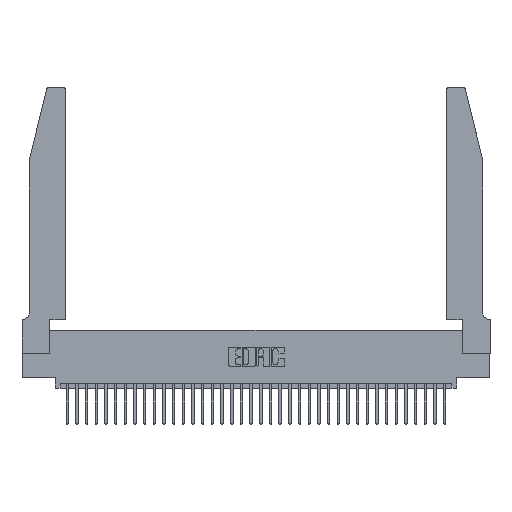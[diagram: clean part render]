
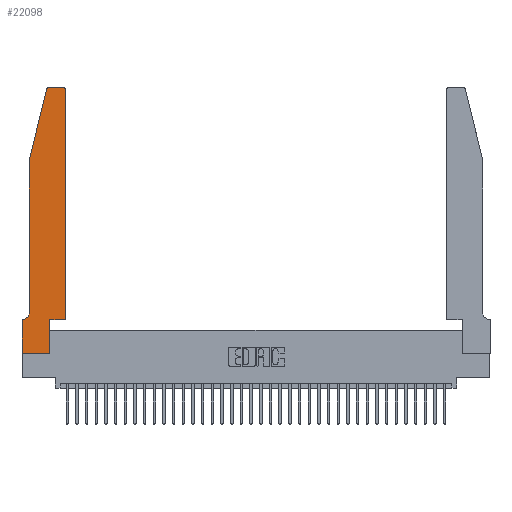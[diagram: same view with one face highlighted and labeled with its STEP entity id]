
A CAD part, top view. The second image highlights one B-rep face of the part: STEP entity #22098.
In plain terms, the highlighted planar face has unit normal (0, 0, 1).
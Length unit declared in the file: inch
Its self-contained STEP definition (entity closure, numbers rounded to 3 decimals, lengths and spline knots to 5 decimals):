
#383 = ORIENTED_EDGE ( 'NONE', *, *, #22573, .T. ) ;
#684 = EDGE_CURVE ( 'NONE', #2675, #20622, #16501, .T. ) ;
#1224 = VERTEX_POINT ( 'NONE', #18128 ) ;
#1583 = EDGE_CURVE ( 'NONE', #23767, #16302, #4445, .T. ) ;
#1666 = DIRECTION ( 'NONE',  ( -1., 0., 0. ) ) ;
#2594 = LINE ( 'NONE', #25634, #26384 ) ;
#2675 = VERTEX_POINT ( 'NONE', #5836 ) ;
#3326 = AXIS2_PLACEMENT_3D ( 'NONE', #4689, #27017, #1666 ) ;
#3863 = CARTESIAN_POINT ( 'NONE',  ( 0., 0.35, 0.37 ) ) ;
#4128 = CARTESIAN_POINT ( 'NONE',  ( 0.0755, 0.35, 0.37 ) ) ;
#4315 = AXIS2_PLACEMENT_3D ( 'NONE', #22122, #36177, #19296 ) ;
#4445 = CIRCLE ( 'NONE', #4315, 0.03 ) ;
#4455 = LINE ( 'NONE', #4128, #26075 ) ;
#4612 = ORIENTED_EDGE ( 'NONE', *, *, #11378, .T. ) ;
#4689 = CARTESIAN_POINT ( 'NONE',  ( 0.0055, 0.42, 0.37 ) ) ;
#5836 = CARTESIAN_POINT ( 'NONE',  ( 0.4505, 0.35, 0.37 ) ) ;
#6321 = DIRECTION ( 'NONE',  ( -0.239, -0.971, 0. ) ) ;
#6413 = ORIENTED_EDGE ( 'NONE', *, *, #23465, .T. ) ;
#6434 = CARTESIAN_POINT ( 'NONE',  ( 0.2865, 0.35, 0.37 ) ) ;
#6522 = EDGE_CURVE ( 'NONE', #20622, #33442, #31228, .T. ) ;
#6792 = CARTESIAN_POINT ( 'NONE',  ( 0.0755, 2., 0.37 ) ) ;
#7374 = LINE ( 'NONE', #18657, #24189 ) ;
#8172 = DIRECTION ( 'NONE',  ( -1., 0., 0. ) ) ;
#8291 = VECTOR ( 'NONE', #10753, 39.37008 ) ;
#9254 = ORIENTED_EDGE ( 'NONE', *, *, #1583, .T. ) ;
#9983 = CARTESIAN_POINT ( 'NONE',  ( 0.4505, 2.72, 0.37 ) ) ;
#10243 = DIRECTION ( 'NONE',  ( 0., 1., 0. ) ) ;
#10327 = DIRECTION ( 'NONE',  ( 1., 0., 0. ) ) ;
#10489 = LINE ( 'NONE', #28172, #11786 ) ;
#10753 = DIRECTION ( 'NONE',  ( 1., 0., 0. ) ) ;
#11176 = PLANE ( 'NONE',  #29555 ) ;
#11275 = VERTEX_POINT ( 'NONE', #21502 ) ;
#11378 = EDGE_CURVE ( 'NONE', #16302, #18760, #2594, .T. ) ;
#11564 = CARTESIAN_POINT ( 'NONE',  ( 0., 0., 0.37 ) ) ;
#11629 = CARTESIAN_POINT ( 'NONE',  ( 0.284, 2.75, 0.37 ) ) ;
#11786 = VECTOR ( 'NONE', #30849, 39.37008 ) ;
#12093 = EDGE_CURVE ( 'NONE', #14893, #27153, #23730, .T. ) ;
#12177 = EDGE_CURVE ( 'NONE', #27153, #2675, #17992, .T. ) ;
#12206 = ORIENTED_EDGE ( 'NONE', *, *, #25421, .T. ) ;
#14321 = ORIENTED_EDGE ( 'NONE', *, *, #12177, .T. ) ;
#14669 = ORIENTED_EDGE ( 'NONE', *, *, #35625, .T. ) ;
#14893 = VERTEX_POINT ( 'NONE', #35311 ) ;
#15030 = ORIENTED_EDGE ( 'NONE', *, *, #19410, .T. ) ;
#16160 = CARTESIAN_POINT ( 'NONE',  ( 0.4505, 0.35, 0.37 ) ) ;
#16302 = VERTEX_POINT ( 'NONE', #30045 ) ;
#16441 = VECTOR ( 'NONE', #31207, 39.37008 ) ;
#16501 = LINE ( 'NONE', #16160, #34468 ) ;
#17051 = CARTESIAN_POINT ( 'NONE',  ( 0.2605, 2.75, 0.37 ) ) ;
#17063 = EDGE_LOOP ( 'NONE', ( #14669, #9254, #4612, #12206, #6413, #383, #15030, #34356, #17687, #14321, #23517, #34891 ) ) ;
#17235 = LINE ( 'NONE', #11564, #16441 ) ;
#17679 = LINE ( 'NONE', #17051, #34008 ) ;
#17687 = ORIENTED_EDGE ( 'NONE', *, *, #12093, .T. ) ;
#17992 = LINE ( 'NONE', #24804, #8291 ) ;
#18128 = CARTESIAN_POINT ( 'NONE',  ( 0., 0., 0.37 ) ) ;
#18170 = FACE_OUTER_BOUND ( 'NONE', #17063, .T. ) ;
#18657 = CARTESIAN_POINT ( 'NONE',  ( 0.0755, 2., 0.37 ) ) ;
#18760 = VERTEX_POINT ( 'NONE', #6792 ) ;
#18912 = CARTESIAN_POINT ( 'NONE',  ( 0.4205, 2.75, 0.37 ) ) ;
#19110 = CARTESIAN_POINT ( 'NONE',  ( 0.4205, 2.72, 0.37 ) ) ;
#19264 = DIRECTION ( 'NONE',  ( 0., 1., 0. ) ) ;
#19296 = DIRECTION ( 'NONE',  ( 1., 0., 0. ) ) ;
#19410 = EDGE_CURVE ( 'NONE', #24110, #1224, #10489, .T. ) ;
#19455 = DIRECTION ( 'NONE',  ( 0., 0., 1. ) ) ;
#20431 = AXIS2_PLACEMENT_3D ( 'NONE', #19110, #32601, #10327 ) ;
#20622 = VERTEX_POINT ( 'NONE', #9983 ) ;
#21502 = CARTESIAN_POINT ( 'NONE',  ( 0.0755, 0.42, 0.37 ) ) ;
#22098 = ADVANCED_FACE ( 'NONE', ( #18170 ), #11176, .T. ) ;
#22122 = CARTESIAN_POINT ( 'NONE',  ( 0.284, 2.72, 0.37 ) ) ;
#22573 = EDGE_CURVE ( 'NONE', #26442, #24110, #4455, .T. ) ;
#22598 = CIRCLE ( 'NONE', #3326, 0.07 ) ;
#23229 = EDGE_CURVE ( 'NONE', #1224, #14893, #17235, .T. ) ;
#23465 = EDGE_CURVE ( 'NONE', #11275, #26442, #22598, .T. ) ;
#23517 = ORIENTED_EDGE ( 'NONE', *, *, #684, .T. ) ;
#23730 = LINE ( 'NONE', #27100, #26775 ) ;
#23767 = VERTEX_POINT ( 'NONE', #11629 ) ;
#23927 = DIRECTION ( 'NONE',  ( -1., 0., 0. ) ) ;
#24110 = VERTEX_POINT ( 'NONE', #3863 ) ;
#24189 = VECTOR ( 'NONE', #24199, 39.37008 ) ;
#24199 = DIRECTION ( 'NONE',  ( 0., -1., 0. ) ) ;
#24804 = CARTESIAN_POINT ( 'NONE',  ( 0.4505, 0.35, 0.37 ) ) ;
#25421 = EDGE_CURVE ( 'NONE', #18760, #11275, #7374, .T. ) ;
#25634 = CARTESIAN_POINT ( 'NONE',  ( 0.0755, 2., 0.37 ) ) ;
#26075 = VECTOR ( 'NONE', #23927, 39.37008 ) ;
#26384 = VECTOR ( 'NONE', #6321, 39.37008 ) ;
#26442 = VERTEX_POINT ( 'NONE', #34064 ) ;
#26775 = VECTOR ( 'NONE', #10243, 39.37008 ) ;
#27017 = DIRECTION ( 'NONE',  ( 0., 0., -1. ) ) ;
#27100 = CARTESIAN_POINT ( 'NONE',  ( 0.2865, 0.35, 0.37 ) ) ;
#27153 = VERTEX_POINT ( 'NONE', #6434 ) ;
#28172 = CARTESIAN_POINT ( 'NONE',  ( 0., 0., 0.37 ) ) ;
#29555 = AXIS2_PLACEMENT_3D ( 'NONE', #36216, #19455, #30713 ) ;
#30045 = CARTESIAN_POINT ( 'NONE',  ( 0.25487, 2.72718, 0.37 ) ) ;
#30713 = DIRECTION ( 'NONE',  ( 1., 0., 0. ) ) ;
#30849 = DIRECTION ( 'NONE',  ( 0., -1., 0. ) ) ;
#31207 = DIRECTION ( 'NONE',  ( 1., 0., 0. ) ) ;
#31228 = CIRCLE ( 'NONE', #20431, 0.03 ) ;
#32601 = DIRECTION ( 'NONE',  ( 0., 0., 1. ) ) ;
#33442 = VERTEX_POINT ( 'NONE', #18912 ) ;
#34008 = VECTOR ( 'NONE', #8172, 39.37008 ) ;
#34064 = CARTESIAN_POINT ( 'NONE',  ( 0.0055, 0.35, 0.37 ) ) ;
#34356 = ORIENTED_EDGE ( 'NONE', *, *, #23229, .T. ) ;
#34468 = VECTOR ( 'NONE', #19264, 39.37008 ) ;
#34891 = ORIENTED_EDGE ( 'NONE', *, *, #6522, .T. ) ;
#35311 = CARTESIAN_POINT ( 'NONE',  ( 0.2865, 0., 0.37 ) ) ;
#35625 = EDGE_CURVE ( 'NONE', #33442, #23767, #17679, .T. ) ;
#36177 = DIRECTION ( 'NONE',  ( 0., 0., 1. ) ) ;
#36216 = CARTESIAN_POINT ( 'NONE',  ( 0., 0.35, 0.37 ) ) ;
